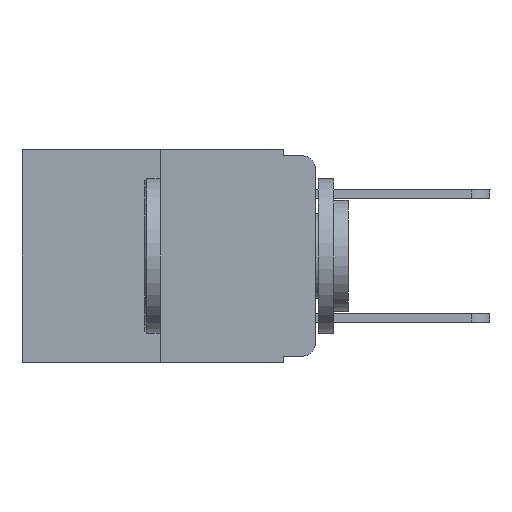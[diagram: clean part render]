
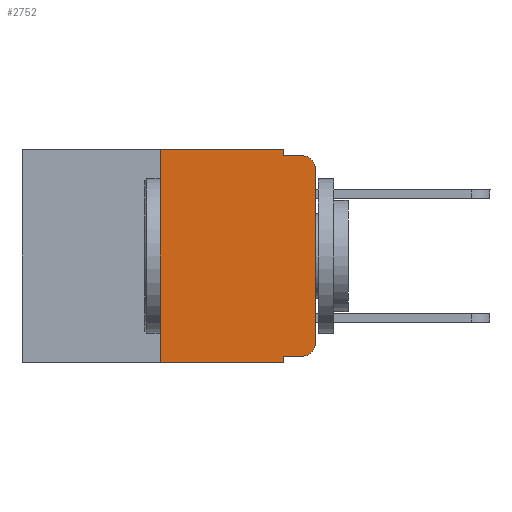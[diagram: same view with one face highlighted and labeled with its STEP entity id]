
A CAD part, left-side view. The second image highlights one B-rep face of the part: STEP entity #2752.
In plain terms, the highlighted planar face has unit normal (-1, 0, 0).
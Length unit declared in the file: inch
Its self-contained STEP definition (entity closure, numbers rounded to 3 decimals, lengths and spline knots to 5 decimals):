
#13 = DIRECTION ( 'NONE',  ( 0., -1., 0. ) ) ;
#113 = DIRECTION ( 'NONE',  ( 0., -1., 0. ) ) ;
#839 = DIRECTION ( 'NONE',  ( 0., -1., 0. ) ) ;
#891 = VERTEX_POINT ( 'NONE', #5992 ) ;
#944 = LINE ( 'NONE', #16560, #15866 ) ;
#1264 = EDGE_CURVE ( 'NONE', #14077, #14705, #15996, .T. ) ;
#1376 = ORIENTED_EDGE ( 'NONE', *, *, #10828, .F. ) ;
#1611 = CARTESIAN_POINT ( 'NONE',  ( 0., 0.051, 0. ) ) ;
#2022 = VECTOR ( 'NONE', #12759, 39.37008 ) ;
#2060 = CARTESIAN_POINT ( 'NONE',  ( 0., 0.051, 0. ) ) ;
#2099 = CARTESIAN_POINT ( 'NONE',  ( 0., 0.051, -0.333 ) ) ;
#2138 = LINE ( 'NONE', #10378, #2022 ) ;
#2700 = ORIENTED_EDGE ( 'NONE', *, *, #5163, .T. ) ;
#2752 = ADVANCED_FACE ( 'NONE', ( #12153 ), #5542, .F. ) ;
#3070 = EDGE_CURVE ( 'NONE', #13104, #14781, #12809, .T. ) ;
#3644 = EDGE_CURVE ( 'NONE', #8790, #13104, #7720, .T. ) ;
#3692 = AXIS2_PLACEMENT_3D ( 'NONE', #11981, #8123, #16005 ) ;
#4056 = CARTESIAN_POINT ( 'NONE',  ( 0., 0.473, -0.343 ) ) ;
#4201 = VERTEX_POINT ( 'NONE', #6500 ) ;
#4322 = DIRECTION ( 'NONE',  ( -1., 0., 0. ) ) ;
#4412 = DIRECTION ( 'NONE',  ( 0., 0., -1. ) ) ;
#4806 = ORIENTED_EDGE ( 'NONE', *, *, #13739, .T. ) ;
#4966 = ORIENTED_EDGE ( 'NONE', *, *, #11098, .T. ) ;
#5163 = EDGE_CURVE ( 'NONE', #4201, #14814, #13239, .T. ) ;
#5414 = CIRCLE ( 'NONE', #9813, 0.02 ) ;
#5542 = PLANE ( 'NONE',  #3692 ) ;
#5992 = CARTESIAN_POINT ( 'NONE',  ( 0., 0.02, -0.333 ) ) ;
#6000 = LINE ( 'NONE', #2060, #8164 ) ;
#6265 = EDGE_LOOP ( 'NONE', ( #8341, #14517, #1376, #9286, #7338, #10349, #2700, #13630, #4806, #4966 ) ) ;
#6500 = CARTESIAN_POINT ( 'NONE',  ( 0., 0.25, -0.343 ) ) ;
#7295 = EDGE_CURVE ( 'NONE', #4201, #8790, #2138, .T. ) ;
#7315 = CARTESIAN_POINT ( 'NONE',  ( 0., 0.051, -0.01 ) ) ;
#7325 = CARTESIAN_POINT ( 'NONE',  ( 0., 0.051, -0.01 ) ) ;
#7338 = ORIENTED_EDGE ( 'NONE', *, *, #3644, .F. ) ;
#7418 = DIRECTION ( 'NONE',  ( 0., 0., -1. ) ) ;
#7648 = VERTEX_POINT ( 'NONE', #2099 ) ;
#7720 = LINE ( 'NONE', #14499, #7945 ) ;
#7945 = VECTOR ( 'NONE', #13, 39.37008 ) ;
#8123 = DIRECTION ( 'NONE',  ( 1., 0., 0. ) ) ;
#8164 = VECTOR ( 'NONE', #16389, 39.37008 ) ;
#8341 = ORIENTED_EDGE ( 'NONE', *, *, #12468, .T. ) ;
#8459 = VECTOR ( 'NONE', #10768, 39.37008 ) ;
#8493 = VERTEX_POINT ( 'NONE', #13481 ) ;
#8723 = CARTESIAN_POINT ( 'NONE',  ( 0., 0.02, -0.01 ) ) ;
#8734 = DIRECTION ( 'NONE',  ( -1., 0., 0. ) ) ;
#8790 = VERTEX_POINT ( 'NONE', #10894 ) ;
#9286 = ORIENTED_EDGE ( 'NONE', *, *, #3070, .F. ) ;
#9486 = CARTESIAN_POINT ( 'NONE',  ( 0., 0.051, -0.333 ) ) ;
#9813 = AXIS2_PLACEMENT_3D ( 'NONE', #16177, #4322, #4412 ) ;
#10349 = ORIENTED_EDGE ( 'NONE', *, *, #7295, .F. ) ;
#10378 = CARTESIAN_POINT ( 'NONE',  ( 0., 0.25, 0. ) ) ;
#10768 = DIRECTION ( 'NONE',  ( 0., -1., 0. ) ) ;
#10828 = EDGE_CURVE ( 'NONE', #14781, #14705, #11377, .T. ) ;
#10894 = CARTESIAN_POINT ( 'NONE',  ( 0., 0.25, 0. ) ) ;
#11098 = EDGE_CURVE ( 'NONE', #891, #8493, #5414, .T. ) ;
#11317 = DIRECTION ( 'NONE',  ( 0., 0., 1. ) ) ;
#11377 = LINE ( 'NONE', #7325, #12258 ) ;
#11444 = DIRECTION ( 'NONE',  ( 0., 0., -1. ) ) ;
#11544 = CARTESIAN_POINT ( 'NONE',  ( 0., 0.051, -0.343 ) ) ;
#11981 = CARTESIAN_POINT ( 'NONE',  ( 0., 0.473, 0. ) ) ;
#12153 = FACE_OUTER_BOUND ( 'NONE', #6265, .T. ) ;
#12258 = VECTOR ( 'NONE', #839, 39.37008 ) ;
#12311 = EDGE_CURVE ( 'NONE', #7648, #14814, #6000, .T. ) ;
#12468 = EDGE_CURVE ( 'NONE', #8493, #14077, #944, .T. ) ;
#12499 = CARTESIAN_POINT ( 'NONE',  ( 0., 0., -0.03 ) ) ;
#12759 = DIRECTION ( 'NONE',  ( 0., 0., 1. ) ) ;
#12809 = LINE ( 'NONE', #14101, #15006 ) ;
#13104 = VERTEX_POINT ( 'NONE', #1611 ) ;
#13239 = LINE ( 'NONE', #4056, #14075 ) ;
#13481 = CARTESIAN_POINT ( 'NONE',  ( 0., 0., -0.313 ) ) ;
#13630 = ORIENTED_EDGE ( 'NONE', *, *, #12311, .F. ) ;
#13653 = LINE ( 'NONE', #9486, #8459 ) ;
#13739 = EDGE_CURVE ( 'NONE', #7648, #891, #13653, .T. ) ;
#14075 = VECTOR ( 'NONE', #113, 39.37008 ) ;
#14077 = VERTEX_POINT ( 'NONE', #12499 ) ;
#14101 = CARTESIAN_POINT ( 'NONE',  ( 0., 0.051, 0. ) ) ;
#14499 = CARTESIAN_POINT ( 'NONE',  ( 0., 0.473, 0. ) ) ;
#14517 = ORIENTED_EDGE ( 'NONE', *, *, #1264, .T. ) ;
#14705 = VERTEX_POINT ( 'NONE', #8723 ) ;
#14781 = VERTEX_POINT ( 'NONE', #7315 ) ;
#14814 = VERTEX_POINT ( 'NONE', #11544 ) ;
#14890 = CARTESIAN_POINT ( 'NONE',  ( 0., 0.02, -0.03 ) ) ;
#15006 = VECTOR ( 'NONE', #11444, 39.37008 ) ;
#15714 = AXIS2_PLACEMENT_3D ( 'NONE', #14890, #8734, #7418 ) ;
#15866 = VECTOR ( 'NONE', #11317, 39.37008 ) ;
#15996 = CIRCLE ( 'NONE', #15714, 0.02 ) ;
#16005 = DIRECTION ( 'NONE',  ( 0., 0., -1. ) ) ;
#16177 = CARTESIAN_POINT ( 'NONE',  ( 0., 0.02, -0.313 ) ) ;
#16389 = DIRECTION ( 'NONE',  ( 0., 0., -1. ) ) ;
#16560 = CARTESIAN_POINT ( 'NONE',  ( 0., 0., 0. ) ) ;
